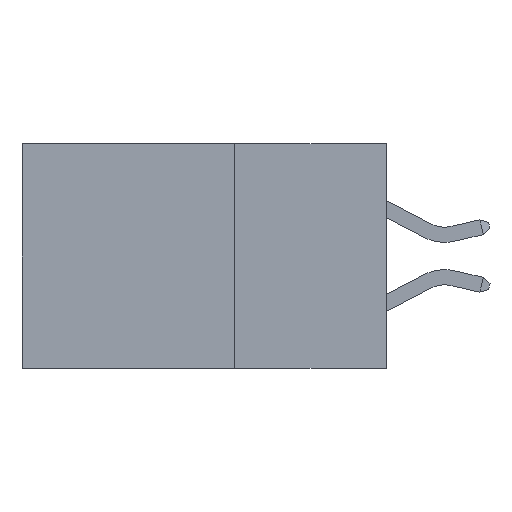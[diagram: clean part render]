
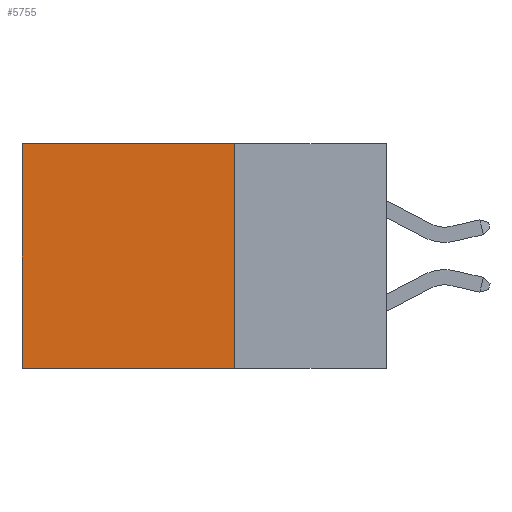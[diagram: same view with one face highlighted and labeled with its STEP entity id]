
A CAD part, left-side view. The second image highlights one B-rep face of the part: STEP entity #5755.
In plain terms, the highlighted planar face has unit normal (-1, 0, 0).
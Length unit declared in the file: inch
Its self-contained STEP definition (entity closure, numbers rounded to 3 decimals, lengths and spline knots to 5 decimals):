
#1219 = DIRECTION ( 'NONE',  ( 1., 0., 0. ) ) ;
#1637 = VERTEX_POINT ( 'NONE', #12381 ) ;
#2805 = FACE_OUTER_BOUND ( 'NONE', #6003, .T. ) ;
#3064 = CARTESIAN_POINT ( 'NONE',  ( 0.2615, 0.25, 0. ) ) ;
#3218 = EDGE_CURVE ( 'NONE', #4015, #1637, #10352, .T. ) ;
#3314 = CARTESIAN_POINT ( 'NONE',  ( 0.2615, 0.25, -0.37 ) ) ;
#3492 = ORIENTED_EDGE ( 'NONE', *, *, #3218, .T. ) ;
#3607 = EDGE_CURVE ( 'NONE', #4015, #5312, #10575, .T. ) ;
#4015 = VERTEX_POINT ( 'NONE', #3064 ) ;
#4637 = VECTOR ( 'NONE', #7885, 39.37008 ) ;
#5257 = CARTESIAN_POINT ( 'NONE',  ( 0.2615, 0.25, -0.37 ) ) ;
#5312 = VERTEX_POINT ( 'NONE', #5257 ) ;
#5732 = ORIENTED_EDGE ( 'NONE', *, *, #7112, .F. ) ;
#5755 = ADVANCED_FACE ( 'NONE', ( #2805 ), #7671, .F. ) ;
#5866 = LINE ( 'NONE', #3314, #13474 ) ;
#6003 = EDGE_LOOP ( 'NONE', ( #7668, #5732, #8819, #3492 ) ) ;
#6270 = CARTESIAN_POINT ( 'NONE',  ( 0.2615, 0.6, -0.37 ) ) ;
#6692 = CARTESIAN_POINT ( 'NONE',  ( 0.2615, 0.25, -0.37 ) ) ;
#6880 = VERTEX_POINT ( 'NONE', #6270 ) ;
#7112 = EDGE_CURVE ( 'NONE', #5312, #6880, #5866, .T. ) ;
#7668 = ORIENTED_EDGE ( 'NONE', *, *, #8939, .T. ) ;
#7671 = PLANE ( 'NONE',  #11734 ) ;
#7885 = DIRECTION ( 'NONE',  ( 0., 0., -1. ) ) ;
#7948 = DIRECTION ( 'NONE',  ( 0., 0., -1. ) ) ;
#7950 = CARTESIAN_POINT ( 'NONE',  ( 0.2615, 0.6, -0.37 ) ) ;
#8111 = VECTOR ( 'NONE', #7948, 39.37008 ) ;
#8244 = CARTESIAN_POINT ( 'NONE',  ( 0.2615, 0.25, -0.37 ) ) ;
#8819 = ORIENTED_EDGE ( 'NONE', *, *, #3607, .F. ) ;
#8939 = EDGE_CURVE ( 'NONE', #1637, #6880, #11274, .T. ) ;
#10011 = VECTOR ( 'NONE', #11807, 39.37008 ) ;
#10352 = LINE ( 'NONE', #11696, #10011 ) ;
#10575 = LINE ( 'NONE', #8244, #4637 ) ;
#10617 = DIRECTION ( 'NONE',  ( 0., 0., -1. ) ) ;
#11274 = LINE ( 'NONE', #7950, #8111 ) ;
#11485 = DIRECTION ( 'NONE',  ( 0., 1., 0. ) ) ;
#11696 = CARTESIAN_POINT ( 'NONE',  ( 0.2615, 0.25, 0. ) ) ;
#11734 = AXIS2_PLACEMENT_3D ( 'NONE', #6692, #1219, #10617 ) ;
#11807 = DIRECTION ( 'NONE',  ( 0., 1., 0. ) ) ;
#12381 = CARTESIAN_POINT ( 'NONE',  ( 0.2615, 0.6, 0. ) ) ;
#13474 = VECTOR ( 'NONE', #11485, 39.37008 ) ;
